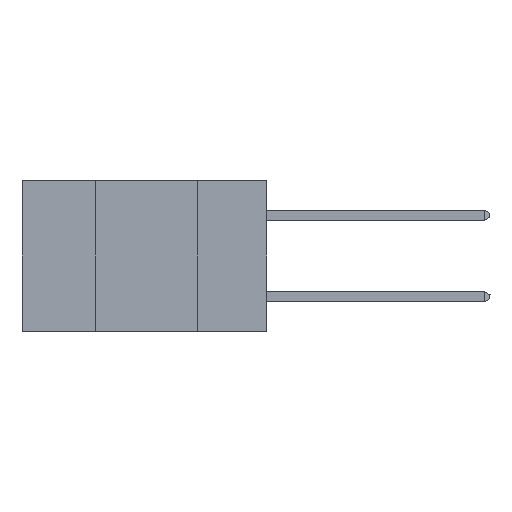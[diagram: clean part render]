
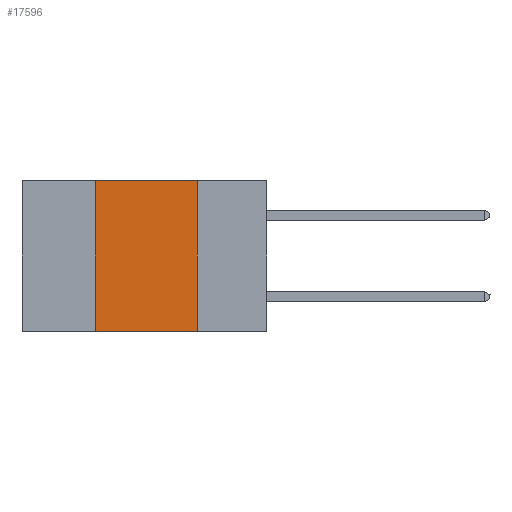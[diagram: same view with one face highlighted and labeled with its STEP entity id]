
A CAD part, left-side view. The second image highlights one B-rep face of the part: STEP entity #17596.
In plain terms, the highlighted planar face has unit normal (-1, 0, 0).
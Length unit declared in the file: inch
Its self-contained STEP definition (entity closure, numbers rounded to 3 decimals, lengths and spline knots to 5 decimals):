
#1742 = CARTESIAN_POINT ( 'NONE',  ( 0., 0.6, 0. ) ) ;
#2365 = DIRECTION ( 'NONE',  ( 1., 0., 0. ) ) ;
#2908 = LINE ( 'NONE', #13819, #8138 ) ;
#2951 = EDGE_CURVE ( 'NONE', #23557, #21086, #22359, .T. ) ;
#4165 = EDGE_CURVE ( 'NONE', #13208, #23557, #8311, .T. ) ;
#4274 = ORIENTED_EDGE ( 'NONE', *, *, #16584, .F. ) ;
#4607 = VECTOR ( 'NONE', #5410, 39.37008 ) ;
#5166 = DIRECTION ( 'NONE',  ( 0., 0., 1. ) ) ;
#5410 = DIRECTION ( 'NONE',  ( 0., -1., 0. ) ) ;
#8138 = VECTOR ( 'NONE', #8316, 39.37008 ) ;
#8311 = LINE ( 'NONE', #23531, #16457 ) ;
#8316 = DIRECTION ( 'NONE',  ( 0., 0., -1. ) ) ;
#8716 = CARTESIAN_POINT ( 'NONE',  ( 0., 0.17, 0. ) ) ;
#10435 = EDGE_CURVE ( 'NONE', #13208, #13098, #15210, .T. ) ;
#11265 = AXIS2_PLACEMENT_3D ( 'NONE', #17476, #2365, #20982 ) ;
#13098 = VERTEX_POINT ( 'NONE', #17965 ) ;
#13208 = VERTEX_POINT ( 'NONE', #23733 ) ;
#13286 = ORIENTED_EDGE ( 'NONE', *, *, #4165, .F. ) ;
#13605 = CARTESIAN_POINT ( 'NONE',  ( 0., 0.6, -0.37 ) ) ;
#13610 = FACE_OUTER_BOUND ( 'NONE', #20514, .T. ) ;
#13720 = PLANE ( 'NONE',  #11265 ) ;
#13819 = CARTESIAN_POINT ( 'NONE',  ( 0., 0.17, 0. ) ) ;
#15210 = LINE ( 'NONE', #13605, #16682 ) ;
#15327 = DIRECTION ( 'NONE',  ( 0., -1., 0. ) ) ;
#16457 = VECTOR ( 'NONE', #5166, 39.37008 ) ;
#16584 = EDGE_CURVE ( 'NONE', #21086, #13098, #2908, .T. ) ;
#16682 = VECTOR ( 'NONE', #15327, 39.37008 ) ;
#17476 = CARTESIAN_POINT ( 'NONE',  ( 0., 0.6, 0. ) ) ;
#17596 = ADVANCED_FACE ( 'NONE', ( #13610 ), #13720, .F. ) ;
#17965 = CARTESIAN_POINT ( 'NONE',  ( 0., 0.17, -0.37 ) ) ;
#20514 = EDGE_LOOP ( 'NONE', ( #4274, #23858, #13286, #21049 ) ) ;
#20982 = DIRECTION ( 'NONE',  ( 0., 0., -1. ) ) ;
#21049 = ORIENTED_EDGE ( 'NONE', *, *, #10435, .T. ) ;
#21086 = VERTEX_POINT ( 'NONE', #8716 ) ;
#21414 = CARTESIAN_POINT ( 'NONE',  ( 0., 0.42, 0. ) ) ;
#22359 = LINE ( 'NONE', #1742, #4607 ) ;
#23531 = CARTESIAN_POINT ( 'NONE',  ( 0., 0.42, 0. ) ) ;
#23557 = VERTEX_POINT ( 'NONE', #21414 ) ;
#23733 = CARTESIAN_POINT ( 'NONE',  ( 0., 0.42, -0.37 ) ) ;
#23858 = ORIENTED_EDGE ( 'NONE', *, *, #2951, .F. ) ;
